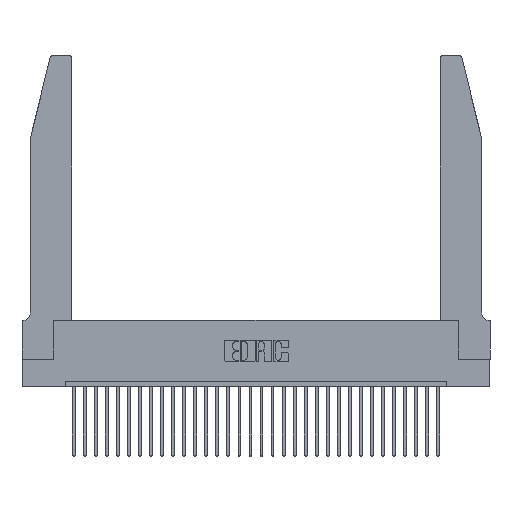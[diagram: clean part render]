
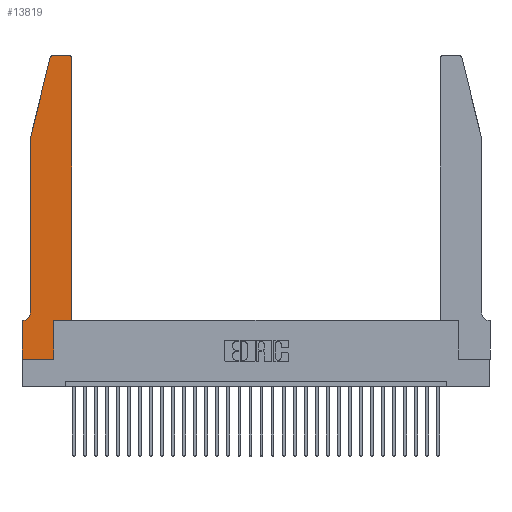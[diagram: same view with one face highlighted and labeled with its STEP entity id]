
A CAD part, top view. The second image highlights one B-rep face of the part: STEP entity #13819.
In plain terms, the highlighted planar face has unit normal (0, 0, 1).
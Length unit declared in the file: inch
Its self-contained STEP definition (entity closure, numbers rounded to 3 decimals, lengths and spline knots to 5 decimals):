
#42 = CARTESIAN_POINT ( 'NONE',  ( 0.4505, 0.35, 0.37 ) ) ;
#71 = LINE ( 'NONE', #7742, #9131 ) ;
#303 = CARTESIAN_POINT ( 'NONE',  ( 0.0755, 0.42, 0.37 ) ) ;
#978 = CARTESIAN_POINT ( 'NONE',  ( 0.25487, 2.72718, 0.37 ) ) ;
#1249 = CARTESIAN_POINT ( 'NONE',  ( 0.284, 2.72, 0.37 ) ) ;
#1358 = AXIS2_PLACEMENT_3D ( 'NONE', #29156, #4631, #28942 ) ;
#1585 = ORIENTED_EDGE ( 'NONE', *, *, #4955, .T. ) ;
#3218 = VECTOR ( 'NONE', #8191, 39.37008 ) ;
#4083 = EDGE_CURVE ( 'NONE', #10360, #30677, #71, .T. ) ;
#4383 = DIRECTION ( 'NONE',  ( 0., -1., 0. ) ) ;
#4631 = DIRECTION ( 'NONE',  ( 0., 0., 1. ) ) ;
#4955 = EDGE_CURVE ( 'NONE', #30677, #16558, #19283, .T. ) ;
#5247 = EDGE_CURVE ( 'NONE', #16558, #15217, #22315, .T. ) ;
#5772 = EDGE_CURVE ( 'NONE', #7099, #15398, #18110, .T. ) ;
#6467 = EDGE_LOOP ( 'NONE', ( #14061, #29963, #29165, #28035, #14553, #17632, #1585, #15273, #10473, #15659, #19670, #18809 ) ) ;
#6487 = EDGE_CURVE ( 'NONE', #25240, #26797, #17273, .T. ) ;
#6988 = DIRECTION ( 'NONE',  ( -1., 0., 0. ) ) ;
#7099 = VERTEX_POINT ( 'NONE', #42 ) ;
#7131 = CARTESIAN_POINT ( 'NONE',  ( 0., 0.35, 0.37 ) ) ;
#7742 = CARTESIAN_POINT ( 'NONE',  ( 0.0755, 0.35, 0.37 ) ) ;
#8191 = DIRECTION ( 'NONE',  ( -0.239, -0.971, 0. ) ) ;
#8330 = AXIS2_PLACEMENT_3D ( 'NONE', #1249, #20670, #30313 ) ;
#9131 = VECTOR ( 'NONE', #12176, 39.37008 ) ;
#9157 = CARTESIAN_POINT ( 'NONE',  ( 0.0755, 2., 0.37 ) ) ;
#9161 = EDGE_CURVE ( 'NONE', #15217, #31061, #20196, .T. ) ;
#9539 = CARTESIAN_POINT ( 'NONE',  ( 0.2605, 2.75, 0.37 ) ) ;
#9823 = VECTOR ( 'NONE', #30790, 39.37008 ) ;
#9842 = EDGE_CURVE ( 'NONE', #15398, #25240, #17471, .T. ) ;
#9852 = VECTOR ( 'NONE', #30952, 39.37008 ) ;
#10360 = VERTEX_POINT ( 'NONE', #19893 ) ;
#10473 = ORIENTED_EDGE ( 'NONE', *, *, #9161, .T. ) ;
#10736 = DIRECTION ( 'NONE',  ( 0., -1., 0. ) ) ;
#11585 = DIRECTION ( 'NONE',  ( 0., 0., 1. ) ) ;
#11731 = EDGE_CURVE ( 'NONE', #27915, #15344, #15599, .T. ) ;
#12176 = DIRECTION ( 'NONE',  ( -1., 0., 0. ) ) ;
#12284 = LINE ( 'NONE', #25311, #3218 ) ;
#12906 = CARTESIAN_POINT ( 'NONE',  ( 0., 0., 0.37 ) ) ;
#13819 = ADVANCED_FACE ( 'NONE', ( #29867 ), #23343, .T. ) ;
#14061 = ORIENTED_EDGE ( 'NONE', *, *, #6487, .T. ) ;
#14073 = CARTESIAN_POINT ( 'NONE',  ( 0.4505, 2.72, 0.37 ) ) ;
#14256 = VECTOR ( 'NONE', #22100, 39.37008 ) ;
#14366 = DIRECTION ( 'NONE',  ( 0., 0., -1. ) ) ;
#14553 = ORIENTED_EDGE ( 'NONE', *, *, #27930, .T. ) ;
#14896 = CARTESIAN_POINT ( 'NONE',  ( 0., 0., 0.37 ) ) ;
#15217 = VERTEX_POINT ( 'NONE', #16749 ) ;
#15273 = ORIENTED_EDGE ( 'NONE', *, *, #5247, .T. ) ;
#15344 = VERTEX_POINT ( 'NONE', #303 ) ;
#15398 = VERTEX_POINT ( 'NONE', #14073 ) ;
#15551 = CARTESIAN_POINT ( 'NONE',  ( 0.0755, 2., 0.37 ) ) ;
#15568 = EDGE_CURVE ( 'NONE', #29729, #27915, #12284, .T. ) ;
#15599 = LINE ( 'NONE', #15551, #23954 ) ;
#15659 = ORIENTED_EDGE ( 'NONE', *, *, #22991, .T. ) ;
#15725 = CIRCLE ( 'NONE', #22565, 0.07 ) ;
#15860 = VECTOR ( 'NONE', #21824, 39.37008 ) ;
#16558 = VERTEX_POINT ( 'NONE', #14896 ) ;
#16632 = CARTESIAN_POINT ( 'NONE',  ( 0.0055, 0.42, 0.37 ) ) ;
#16749 = CARTESIAN_POINT ( 'NONE',  ( 0.2865, 0., 0.37 ) ) ;
#17273 = LINE ( 'NONE', #9539, #29425 ) ;
#17471 = CIRCLE ( 'NONE', #1358, 0.03 ) ;
#17632 = ORIENTED_EDGE ( 'NONE', *, *, #4083, .T. ) ;
#18110 = LINE ( 'NONE', #21894, #14256 ) ;
#18537 = VECTOR ( 'NONE', #4383, 39.37008 ) ;
#18809 = ORIENTED_EDGE ( 'NONE', *, *, #9842, .T. ) ;
#18994 = LINE ( 'NONE', #23483, #9823 ) ;
#19283 = LINE ( 'NONE', #12906, #18537 ) ;
#19360 = CARTESIAN_POINT ( 'NONE',  ( 0.284, 2.75, 0.37 ) ) ;
#19670 = ORIENTED_EDGE ( 'NONE', *, *, #5772, .T. ) ;
#19782 = CIRCLE ( 'NONE', #8330, 0.03 ) ;
#19893 = CARTESIAN_POINT ( 'NONE',  ( 0.0055, 0.35, 0.37 ) ) ;
#20196 = LINE ( 'NONE', #28606, #9852 ) ;
#20670 = DIRECTION ( 'NONE',  ( 0., 0., 1. ) ) ;
#21824 = DIRECTION ( 'NONE',  ( 1., 0., 0. ) ) ;
#21894 = CARTESIAN_POINT ( 'NONE',  ( 0.4505, 0.35, 0.37 ) ) ;
#22100 = DIRECTION ( 'NONE',  ( 0., 1., 0. ) ) ;
#22315 = LINE ( 'NONE', #29017, #15860 ) ;
#22565 = AXIS2_PLACEMENT_3D ( 'NONE', #16632, #14366, #31266 ) ;
#22991 = EDGE_CURVE ( 'NONE', #31061, #7099, #18994, .T. ) ;
#23343 = PLANE ( 'NONE',  #29102 ) ;
#23483 = CARTESIAN_POINT ( 'NONE',  ( 0.4505, 0.35, 0.37 ) ) ;
#23954 = VECTOR ( 'NONE', #10736, 39.37008 ) ;
#25240 = VERTEX_POINT ( 'NONE', #26907 ) ;
#25311 = CARTESIAN_POINT ( 'NONE',  ( 0.0755, 2., 0.37 ) ) ;
#26797 = VERTEX_POINT ( 'NONE', #19360 ) ;
#26907 = CARTESIAN_POINT ( 'NONE',  ( 0.4205, 2.75, 0.37 ) ) ;
#27299 = CARTESIAN_POINT ( 'NONE',  ( 0.2865, 0.35, 0.37 ) ) ;
#27915 = VERTEX_POINT ( 'NONE', #9157 ) ;
#27930 = EDGE_CURVE ( 'NONE', #15344, #10360, #15725, .T. ) ;
#28035 = ORIENTED_EDGE ( 'NONE', *, *, #11731, .T. ) ;
#28606 = CARTESIAN_POINT ( 'NONE',  ( 0.2865, 0.35, 0.37 ) ) ;
#28942 = DIRECTION ( 'NONE',  ( 1., 0., 0. ) ) ;
#29017 = CARTESIAN_POINT ( 'NONE',  ( 0., 0., 0.37 ) ) ;
#29102 = AXIS2_PLACEMENT_3D ( 'NONE', #7131, #11585, #31058 ) ;
#29156 = CARTESIAN_POINT ( 'NONE',  ( 0.4205, 2.72, 0.37 ) ) ;
#29165 = ORIENTED_EDGE ( 'NONE', *, *, #15568, .T. ) ;
#29425 = VECTOR ( 'NONE', #6988, 39.37008 ) ;
#29729 = VERTEX_POINT ( 'NONE', #978 ) ;
#29867 = FACE_OUTER_BOUND ( 'NONE', #6467, .T. ) ;
#29963 = ORIENTED_EDGE ( 'NONE', *, *, #30500, .T. ) ;
#30313 = DIRECTION ( 'NONE',  ( 1., 0., 0. ) ) ;
#30500 = EDGE_CURVE ( 'NONE', #26797, #29729, #19782, .T. ) ;
#30518 = CARTESIAN_POINT ( 'NONE',  ( 0., 0.35, 0.37 ) ) ;
#30677 = VERTEX_POINT ( 'NONE', #30518 ) ;
#30790 = DIRECTION ( 'NONE',  ( 1., 0., 0. ) ) ;
#30952 = DIRECTION ( 'NONE',  ( 0., 1., 0. ) ) ;
#31058 = DIRECTION ( 'NONE',  ( 1., 0., 0. ) ) ;
#31061 = VERTEX_POINT ( 'NONE', #27299 ) ;
#31266 = DIRECTION ( 'NONE',  ( -1., 0., 0. ) ) ;
